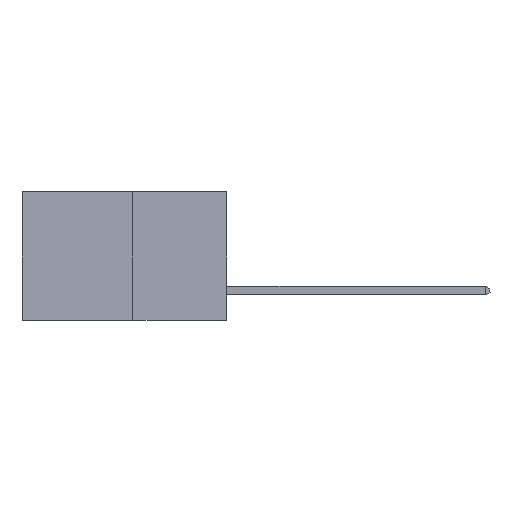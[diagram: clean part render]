
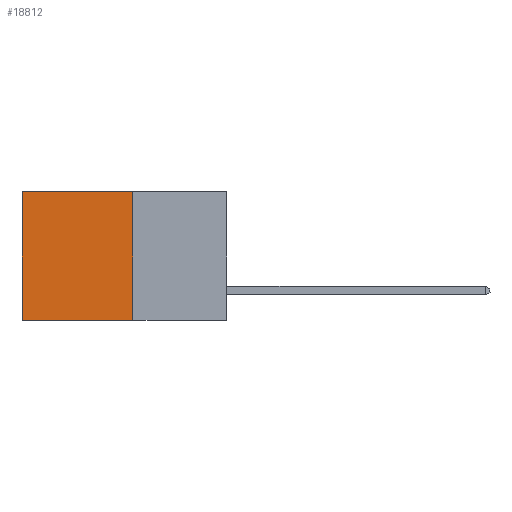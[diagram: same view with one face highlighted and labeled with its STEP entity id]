
A CAD part, left-side view. The second image highlights one B-rep face of the part: STEP entity #18812.
In plain terms, the highlighted planar face has unit normal (-1, 0, 0).
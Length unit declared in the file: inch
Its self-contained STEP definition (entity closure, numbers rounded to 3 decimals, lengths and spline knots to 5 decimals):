
#227 = VECTOR ( 'NONE', #13460, 39.37008 ) ;
#1048 = CARTESIAN_POINT ( 'NONE',  ( 0.277, 0.27, -0.37 ) ) ;
#1260 = VECTOR ( 'NONE', #13053, 39.37008 ) ;
#1299 = PLANE ( 'NONE',  #3065 ) ;
#1358 = DIRECTION ( 'NONE',  ( 0., 0., -1. ) ) ;
#2280 = CARTESIAN_POINT ( 'NONE',  ( 0.277, 0.59, -0.37 ) ) ;
#2646 = DIRECTION ( 'NONE',  ( 0., 0., -1. ) ) ;
#3065 = AXIS2_PLACEMENT_3D ( 'NONE', #19061, #10356, #1358 ) ;
#3280 = CARTESIAN_POINT ( 'NONE',  ( 0.277, 0.27, -0.37 ) ) ;
#4242 = EDGE_CURVE ( 'NONE', #4611, #13313, #4288, .T. ) ;
#4283 = ORIENTED_EDGE ( 'NONE', *, *, #7458, .T. ) ;
#4288 = LINE ( 'NONE', #3280, #17691 ) ;
#4611 = VERTEX_POINT ( 'NONE', #11178 ) ;
#4843 = LINE ( 'NONE', #2280, #16218 ) ;
#5478 = ORIENTED_EDGE ( 'NONE', *, *, #4242, .F. ) ;
#5598 = EDGE_CURVE ( 'NONE', #4611, #18862, #5634, .T. ) ;
#5634 = LINE ( 'NONE', #13722, #227 ) ;
#5769 = LINE ( 'NONE', #1048, #1260 ) ;
#5771 = ORIENTED_EDGE ( 'NONE', *, *, #5598, .T. ) ;
#7458 = EDGE_CURVE ( 'NONE', #18862, #11550, #4843, .T. ) ;
#10356 = DIRECTION ( 'NONE',  ( 1., 0., 0. ) ) ;
#11178 = CARTESIAN_POINT ( 'NONE',  ( 0.277, 0.27, 0. ) ) ;
#11550 = VERTEX_POINT ( 'NONE', #16603 ) ;
#11817 = CARTESIAN_POINT ( 'NONE',  ( 0.277, 0.27, -0.37 ) ) ;
#13053 = DIRECTION ( 'NONE',  ( 0., 1., 0. ) ) ;
#13313 = VERTEX_POINT ( 'NONE', #11817 ) ;
#13460 = DIRECTION ( 'NONE',  ( 0., 1., 0. ) ) ;
#13722 = CARTESIAN_POINT ( 'NONE',  ( 0.277, 0.27, 0. ) ) ;
#14498 = DIRECTION ( 'NONE',  ( 0., 0., -1. ) ) ;
#16218 = VECTOR ( 'NONE', #2646, 39.37008 ) ;
#16345 = CARTESIAN_POINT ( 'NONE',  ( 0.277, 0.59, 0. ) ) ;
#16603 = CARTESIAN_POINT ( 'NONE',  ( 0.277, 0.59, -0.37 ) ) ;
#17164 = EDGE_LOOP ( 'NONE', ( #4283, #17694, #5478, #5771 ) ) ;
#17691 = VECTOR ( 'NONE', #14498, 39.37008 ) ;
#17694 = ORIENTED_EDGE ( 'NONE', *, *, #18657, .F. ) ;
#18174 = FACE_OUTER_BOUND ( 'NONE', #17164, .T. ) ;
#18657 = EDGE_CURVE ( 'NONE', #13313, #11550, #5769, .T. ) ;
#18812 = ADVANCED_FACE ( 'NONE', ( #18174 ), #1299, .F. ) ;
#18862 = VERTEX_POINT ( 'NONE', #16345 ) ;
#19061 = CARTESIAN_POINT ( 'NONE',  ( 0.277, 0.27, -0.37 ) ) ;
